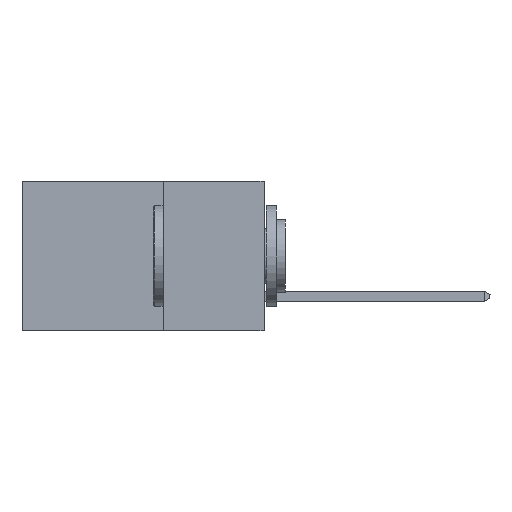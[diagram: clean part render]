
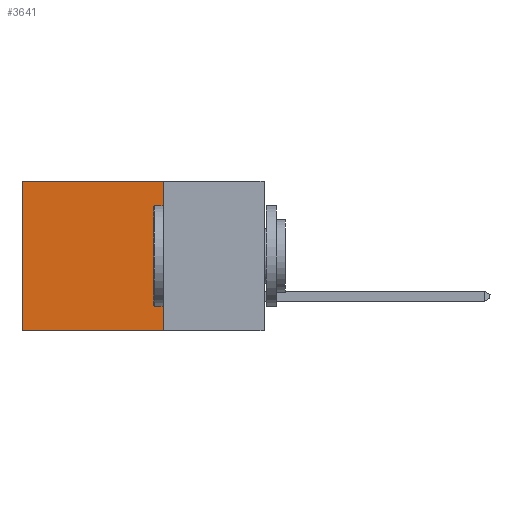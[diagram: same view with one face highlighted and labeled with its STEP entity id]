
A CAD part, left-side view. The second image highlights one B-rep face of the part: STEP entity #3641.
In plain terms, the highlighted planar face has unit normal (-1, 0, 0).
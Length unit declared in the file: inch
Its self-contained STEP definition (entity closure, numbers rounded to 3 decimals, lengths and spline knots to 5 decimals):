
#368 = CARTESIAN_POINT ( 'NONE',  ( 0.2615, 0.6, -0.37 ) ) ;
#830 = CARTESIAN_POINT ( 'NONE',  ( 0.2615, 0.25, -0.37 ) ) ;
#1514 = EDGE_CURVE ( 'NONE', #12989, #4247, #10170, .T. ) ;
#1848 = CARTESIAN_POINT ( 'NONE',  ( 0.2615, 0.25, -0.37 ) ) ;
#2097 = DIRECTION ( 'NONE',  ( 1., 0., 0. ) ) ;
#3249 = VECTOR ( 'NONE', #8421, 39.37008 ) ;
#3379 = VECTOR ( 'NONE', #12888, 39.37008 ) ;
#3625 = AXIS2_PLACEMENT_3D ( 'NONE', #1848, #2097, #10681 ) ;
#3641 = ADVANCED_FACE ( 'NONE', ( #13611 ), #5719, .F. ) ;
#3730 = CARTESIAN_POINT ( 'NONE',  ( 0.2615, 0.25, -0.37 ) ) ;
#3945 = ORIENTED_EDGE ( 'NONE', *, *, #4694, .F. ) ;
#4021 = VECTOR ( 'NONE', #8032, 39.37008 ) ;
#4247 = VERTEX_POINT ( 'NONE', #3730 ) ;
#4694 = EDGE_CURVE ( 'NONE', #4247, #12739, #11278, .T. ) ;
#5304 = EDGE_CURVE ( 'NONE', #12989, #7379, #17930, .T. ) ;
#5321 = DIRECTION ( 'NONE',  ( 0., 1., 0. ) ) ;
#5719 = PLANE ( 'NONE',  #3625 ) ;
#5832 = LINE ( 'NONE', #21863, #3379 ) ;
#7245 = CARTESIAN_POINT ( 'NONE',  ( 0.2615, 0.25, 0. ) ) ;
#7379 = VERTEX_POINT ( 'NONE', #16735 ) ;
#7774 = EDGE_CURVE ( 'NONE', #7379, #12739, #5832, .T. ) ;
#8032 = DIRECTION ( 'NONE',  ( 0., 1., 0. ) ) ;
#8421 = DIRECTION ( 'NONE',  ( 0., 0., -1. ) ) ;
#8539 = CARTESIAN_POINT ( 'NONE',  ( 0.2615, 0.25, -0.37 ) ) ;
#10170 = LINE ( 'NONE', #8539, #3249 ) ;
#10681 = DIRECTION ( 'NONE',  ( 0., 0., -1. ) ) ;
#10881 = EDGE_LOOP ( 'NONE', ( #12969, #3945, #12285, #11325 ) ) ;
#11278 = LINE ( 'NONE', #830, #4021 ) ;
#11325 = ORIENTED_EDGE ( 'NONE', *, *, #5304, .T. ) ;
#12285 = ORIENTED_EDGE ( 'NONE', *, *, #1514, .F. ) ;
#12739 = VERTEX_POINT ( 'NONE', #368 ) ;
#12888 = DIRECTION ( 'NONE',  ( 0., 0., -1. ) ) ;
#12969 = ORIENTED_EDGE ( 'NONE', *, *, #7774, .T. ) ;
#12989 = VERTEX_POINT ( 'NONE', #22471 ) ;
#13611 = FACE_OUTER_BOUND ( 'NONE', #10881, .T. ) ;
#14049 = VECTOR ( 'NONE', #5321, 39.37008 ) ;
#16735 = CARTESIAN_POINT ( 'NONE',  ( 0.2615, 0.6, 0. ) ) ;
#17930 = LINE ( 'NONE', #7245, #14049 ) ;
#21863 = CARTESIAN_POINT ( 'NONE',  ( 0.2615, 0.6, -0.37 ) ) ;
#22471 = CARTESIAN_POINT ( 'NONE',  ( 0.2615, 0.25, 0. ) ) ;
